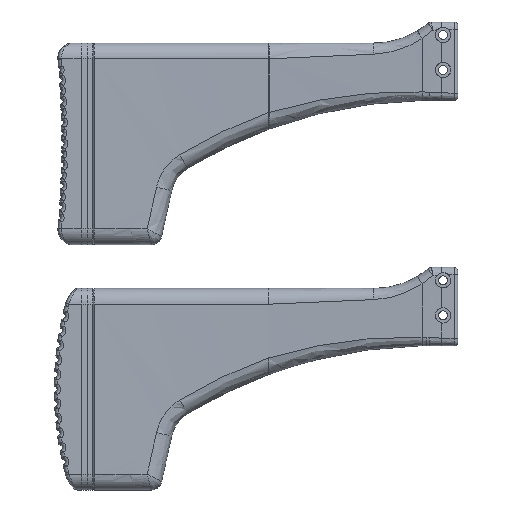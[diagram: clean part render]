
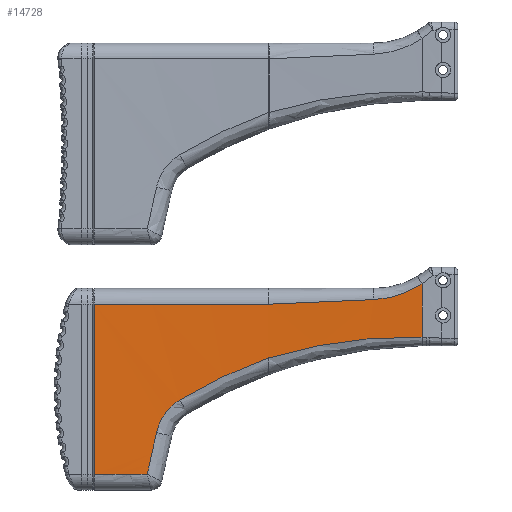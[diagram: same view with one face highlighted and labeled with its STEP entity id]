
A CAD part, left-side view. The second image highlights one B-rep face of the part: STEP entity #14728.
In plain terms, the highlighted cylindrical face has radius 3182.51 mm (diameter 6365.01 mm), a partial arc.
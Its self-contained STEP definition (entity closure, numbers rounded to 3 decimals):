
#90=ELLIPSE('',#16147,14630.042,3182.507);
#320=CYLINDRICAL_SURFACE('',#16144,3182.507);
#818=LINE('',#37126,#1523);
#819=LINE('',#37257,#1524);
#820=LINE('',#37273,#1525);
#1523=VECTOR('',#19188,281.);
#1524=VECTOR('',#19193,10.);
#1525=VECTOR('',#19198,10.);
#2915=FACE_OUTER_BOUND('',#3919,.T.);
#3919=EDGE_LOOP('',(#12308,#12309,#12310,#12311,#12312,#12313,#12314,#12315,
#12316,#12317,#12318,#12319,#12320));
#4664=B_SPLINE_CURVE_WITH_KNOTS('',3,(#37208,#37209,#37210,#37211,#37212),
 .UNSPECIFIED.,.F.,.F.,(4,1,4),(1.162,2.63,3.898),
 .UNSPECIFIED.);
#4665=B_SPLINE_CURVE_WITH_KNOTS('',3,(#37213,#37214,#37215,#37216),
 .UNSPECIFIED.,.F.,.F.,(4,4),(0.939,1.162),
 .UNSPECIFIED.);
#4669=B_SPLINE_CURVE_WITH_KNOTS('',3,(#37241,#37242,#37243,#37244),
 .UNSPECIFIED.,.F.,.F.,(4,4),(0.329,9.059),
 .UNSPECIFIED.);
#4670=B_SPLINE_CURVE_WITH_KNOTS('',3,(#37245,#37246,#37247,#37248),
 .UNSPECIFIED.,.F.,.F.,(4,4),(9.059,9.247),
 .UNSPECIFIED.);
#4671=B_SPLINE_CURVE_WITH_KNOTS('',3,(#37250,#37251,#37252,#37253),
 .UNSPECIFIED.,.F.,.F.,(4,4),(3.898,9.923),
 .UNSPECIFIED.);
#4672=B_SPLINE_CURVE_WITH_KNOTS('',3,(#37263,#37264,#37265,#37266,#37267),
 .UNSPECIFIED.,.F.,.F.,(4,1,4),(0.,0.999,2.331),
 .UNSPECIFIED.);
#4673=B_SPLINE_CURVE_WITH_KNOTS('',3,(#37269,#37270,#37271,#37272),
 .UNSPECIFIED.,.F.,.F.,(4,4),(0.,5.636),
 .UNSPECIFIED.);
#5521=CIRCLE('',#16145,3182.507);
#5522=CIRCLE('',#16146,3182.507);
#6540=VERTEX_POINT('',#37120);
#6541=VERTEX_POINT('',#37125);
#6543=VERTEX_POINT('',#37206);
#6544=VERTEX_POINT('',#37207);
#6547=VERTEX_POINT('',#37239);
#6548=VERTEX_POINT('',#37240);
#6549=VERTEX_POINT('',#37249);
#6550=VERTEX_POINT('',#37254);
#6551=VERTEX_POINT('',#37256);
#6552=VERTEX_POINT('',#37258);
#6553=VERTEX_POINT('',#37260);
#6554=VERTEX_POINT('',#37262);
#6555=VERTEX_POINT('',#37268);
#8521=EDGE_CURVE('',#6541,#6540,#818,.T.);
#8525=EDGE_CURVE('',#6543,#6544,#4664,.T.);
#8526=EDGE_CURVE('',#6540,#6543,#4665,.T.);
#8530=EDGE_CURVE('',#6547,#6548,#4669,.T.);
#8531=EDGE_CURVE('',#6548,#6541,#4670,.T.);
#8532=EDGE_CURVE('',#6544,#6549,#4671,.T.);
#8533=EDGE_CURVE('',#6549,#6550,#5521,.T.);
#8534=EDGE_CURVE('',#6550,#6551,#819,.T.);
#8535=EDGE_CURVE('',#6551,#6552,#5522,.T.);
#8536=EDGE_CURVE('',#6552,#6553,#90,.T.);
#8537=EDGE_CURVE('',#6553,#6554,#4672,.T.);
#8538=EDGE_CURVE('',#6554,#6555,#4673,.T.);
#8539=EDGE_CURVE('',#6555,#6547,#820,.T.);
#12308=ORIENTED_EDGE('',*,*,#8530,.T.);
#12309=ORIENTED_EDGE('',*,*,#8531,.T.);
#12310=ORIENTED_EDGE('',*,*,#8521,.T.);
#12311=ORIENTED_EDGE('',*,*,#8526,.T.);
#12312=ORIENTED_EDGE('',*,*,#8525,.T.);
#12313=ORIENTED_EDGE('',*,*,#8532,.T.);
#12314=ORIENTED_EDGE('',*,*,#8533,.T.);
#12315=ORIENTED_EDGE('',*,*,#8534,.T.);
#12316=ORIENTED_EDGE('',*,*,#8535,.T.);
#12317=ORIENTED_EDGE('',*,*,#8536,.T.);
#12318=ORIENTED_EDGE('',*,*,#8537,.T.);
#12319=ORIENTED_EDGE('',*,*,#8538,.T.);
#12320=ORIENTED_EDGE('',*,*,#8539,.T.);
#14728=ADVANCED_FACE('',(#2915),#320,.F.);
#16144=AXIS2_PLACEMENT_3D('',#37238,#19189,#19190);
#16145=AXIS2_PLACEMENT_3D('',#37255,#19191,#19192);
#16146=AXIS2_PLACEMENT_3D('',#37259,#19194,#19195);
#16147=AXIS2_PLACEMENT_3D('',#37261,#19196,#19197);
#19188=DIRECTION('',(0.,0.,1.));
#19189=DIRECTION('center_axis',(0.,0.,1.));
#19190=DIRECTION('ref_axis',(1.,0.021,0.));
#19191=DIRECTION('center_axis',(0.,0.,1.));
#19192=DIRECTION('ref_axis',(1.,0.004,0.));
#19193=DIRECTION('',(0.,0.,-1.));
#19194=DIRECTION('center_axis',(0.,0.,-1.));
#19195=DIRECTION('ref_axis',(1.,0.015,0.));
#19196=DIRECTION('center_axis',(0.,-0.976,
-0.218));
#19197=DIRECTION('ref_axis',(0.,0.218,-0.976));
#19198=DIRECTION('',(0.,0.,-1.));
#37120=CARTESIAN_POINT('',(-1.304,212.319,-257.936));
#37125=CARTESIAN_POINT('',(-1.304,212.319,-288.474));
#37126=CARTESIAN_POINT('',(-1.304,212.319,-248.588));
#37206=CARTESIAN_POINT('',(-1.23,214.194,-259.134));
#37207=CARTESIAN_POINT('',(-0.33,240.019,-266.981));
#37208=CARTESIAN_POINT('Ctrl Pts',(-1.23,214.194,-259.134));
#37209=CARTESIAN_POINT('Ctrl Pts',(-1.068,218.36,-261.676));
#37210=CARTESIAN_POINT('Ctrl Pts',(-0.756,226.772,
-265.348));
#37211=CARTESIAN_POINT('Ctrl Pts',(-0.459,235.809,
-266.798));
#37212=CARTESIAN_POINT('Ctrl Pts',(-0.33,240.019,-266.981));
#37213=CARTESIAN_POINT('Ctrl Pts',(-1.304,212.319,-257.936));
#37214=CARTESIAN_POINT('Ctrl Pts',(-1.28,212.936,-258.348));
#37215=CARTESIAN_POINT('Ctrl Pts',(-1.255,213.561,-258.748));
#37216=CARTESIAN_POINT('Ctrl Pts',(-1.23,214.194,-259.134));
#37238=CARTESIAN_POINT('Origin',(-3181.326,338.055,-248.588));
#37239=CARTESIAN_POINT('',(0.953,300.,-300.349));
#37240=CARTESIAN_POINT('',(-1.23,214.194,-288.426));
#37241=CARTESIAN_POINT('Ctrl Pts',(0.954,300.001,-300.348));
#37242=CARTESIAN_POINT('Ctrl Pts',(0.625,272.282,-291.823));
#37243=CARTESIAN_POINT('Ctrl Pts',(-0.102,243.19,
-287.779));
#37244=CARTESIAN_POINT('Ctrl Pts',(-1.23,214.194,-288.426));
#37245=CARTESIAN_POINT('Ctrl Pts',(-1.23,214.194,-288.426));
#37246=CARTESIAN_POINT('Ctrl Pts',(-1.255,213.569,-288.44));
#37247=CARTESIAN_POINT('Ctrl Pts',(-1.279,212.944,-288.456));
#37248=CARTESIAN_POINT('Ctrl Pts',(-1.304,212.319,-288.474));
#37249=CARTESIAN_POINT('',(0.953,300.,-269.588));
#37250=CARTESIAN_POINT('Ctrl Pts',(-0.33,240.019,-266.981));
#37251=CARTESIAN_POINT('Ctrl Pts',(0.287,260.02,-267.85));
#37252=CARTESIAN_POINT('Ctrl Pts',(0.714,280.007,-268.719));
#37253=CARTESIAN_POINT('Ctrl Pts',(0.953,300.,-269.588));
#37254=CARTESIAN_POINT('',(0.589,399.4,-269.588));
#37255=CARTESIAN_POINT('Origin',(-3181.326,338.055,-269.588));
#37256=CARTESIAN_POINT('',(0.589,399.4,-366.588));
#37257=CARTESIAN_POINT('',(0.589,399.4,-248.588));
#37258=CARTESIAN_POINT('',(1.029,369.123,-366.588));
#37259=CARTESIAN_POINT('Origin',(-3181.326,338.055,-366.588));
#37260=CARTESIAN_POINT('',(1.076,363.826,-342.825));
#37261=CARTESIAN_POINT('Origin',(-3181.326,338.055,-227.191));
#37262=CARTESIAN_POINT('',(1.156,350.652,-324.385));
#37263=CARTESIAN_POINT('Ctrl Pts',(1.076,363.826,-342.825));
#37264=CARTESIAN_POINT('Ctrl Pts',(1.082,363.102,-339.575));
#37265=CARTESIAN_POINT('Ctrl Pts',(1.106,360.099,-332.286));
#37266=CARTESIAN_POINT('Ctrl Pts',(1.141,354.432,-326.695));
#37267=CARTESIAN_POINT('Ctrl Pts',(1.156,350.652,-324.385));
#37268=CARTESIAN_POINT('',(0.953,300.,-300.194));
#37269=CARTESIAN_POINT('Ctrl Pts',(1.156,350.652,-324.385));
#37270=CARTESIAN_POINT('Ctrl Pts',(1.219,334.654,-314.61));
#37271=CARTESIAN_POINT('Ctrl Pts',(1.164,317.65,-306.489));
#37272=CARTESIAN_POINT('Ctrl Pts',(0.953,300.,-300.194));
#37273=CARTESIAN_POINT('',(0.953,300.,-248.588));
